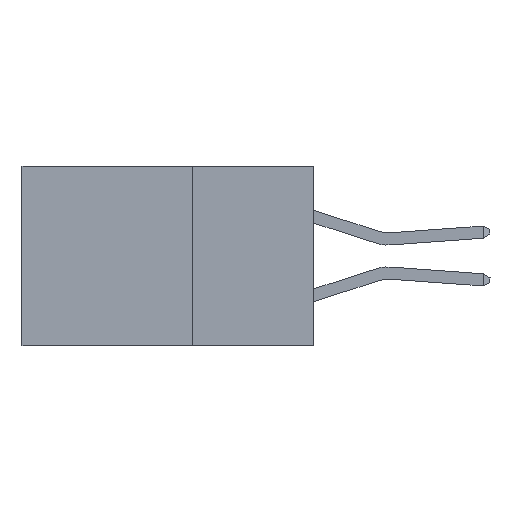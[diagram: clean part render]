
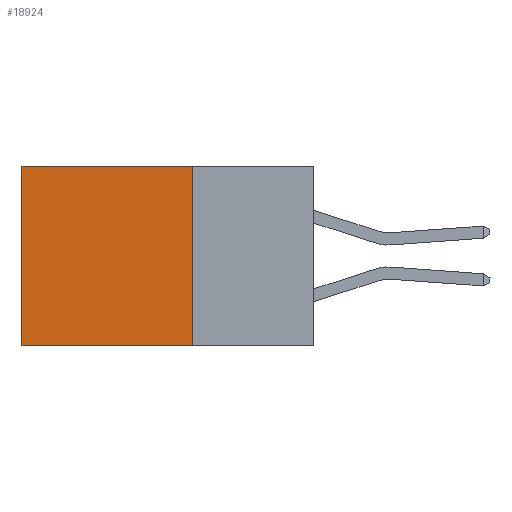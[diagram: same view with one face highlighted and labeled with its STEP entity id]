
A CAD part, left-side view. The second image highlights one B-rep face of the part: STEP entity #18924.
In plain terms, the highlighted planar face has unit normal (-1, 0, 0).
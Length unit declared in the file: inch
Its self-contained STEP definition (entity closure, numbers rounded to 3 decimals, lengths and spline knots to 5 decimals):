
#775 = AXIS2_PLACEMENT_3D ( 'NONE', #8602, #14316, #33722 ) ;
#1108 = DIRECTION ( 'NONE',  ( 0., 1., 0. ) ) ;
#1432 = DIRECTION ( 'NONE',  ( 0., 1., 0. ) ) ;
#2218 = CARTESIAN_POINT ( 'NONE',  ( 0.2875, 0.6, -0.37 ) ) ;
#3618 = EDGE_LOOP ( 'NONE', ( #16414, #12874, #23667, #35190 ) ) ;
#3880 = LINE ( 'NONE', #35024, #18098 ) ;
#6759 = CARTESIAN_POINT ( 'NONE',  ( 0.2875, 0.25, 0. ) ) ;
#6912 = DIRECTION ( 'NONE',  ( 0., 0., -1. ) ) ;
#7972 = CARTESIAN_POINT ( 'NONE',  ( 0.2875, 0.25, -0.37 ) ) ;
#8224 = EDGE_CURVE ( 'NONE', #12353, #23973, #3880, .T. ) ;
#8504 = VECTOR ( 'NONE', #16162, 39.37008 ) ;
#8600 = VECTOR ( 'NONE', #6912, 39.37008 ) ;
#8602 = CARTESIAN_POINT ( 'NONE',  ( 0.2875, 0.25, 0. ) ) ;
#11450 = PLANE ( 'NONE',  #775 ) ;
#12353 = VERTEX_POINT ( 'NONE', #7972 ) ;
#12874 = ORIENTED_EDGE ( 'NONE', *, *, #8224, .F. ) ;
#13288 = CARTESIAN_POINT ( 'NONE',  ( 0.2875, 0.6, 0. ) ) ;
#14132 = VERTEX_POINT ( 'NONE', #25721 ) ;
#14316 = DIRECTION ( 'NONE',  ( 1., 0., 0. ) ) ;
#16162 = DIRECTION ( 'NONE',  ( 0., 0., -1. ) ) ;
#16414 = ORIENTED_EDGE ( 'NONE', *, *, #19381, .T. ) ;
#18098 = VECTOR ( 'NONE', #1432, 39.37008 ) ;
#18575 = VECTOR ( 'NONE', #1108, 39.37008 ) ;
#18924 = ADVANCED_FACE ( 'NONE', ( #24309 ), #11450, .F. ) ;
#19381 = EDGE_CURVE ( 'NONE', #14132, #23973, #24277, .T. ) ;
#23069 = EDGE_CURVE ( 'NONE', #29782, #12353, #31737, .T. ) ;
#23667 = ORIENTED_EDGE ( 'NONE', *, *, #23069, .F. ) ;
#23973 = VERTEX_POINT ( 'NONE', #2218 ) ;
#23997 = CARTESIAN_POINT ( 'NONE',  ( 0.2875, 0.25, 0. ) ) ;
#24277 = LINE ( 'NONE', #13288, #8504 ) ;
#24309 = FACE_OUTER_BOUND ( 'NONE', #3618, .T. ) ;
#25721 = CARTESIAN_POINT ( 'NONE',  ( 0.2875, 0.6, 0. ) ) ;
#25912 = LINE ( 'NONE', #6759, #18575 ) ;
#29209 = CARTESIAN_POINT ( 'NONE',  ( 0.2875, 0.25, 0. ) ) ;
#29782 = VERTEX_POINT ( 'NONE', #23997 ) ;
#31737 = LINE ( 'NONE', #29209, #8600 ) ;
#33510 = EDGE_CURVE ( 'NONE', #29782, #14132, #25912, .T. ) ;
#33722 = DIRECTION ( 'NONE',  ( 0., 0., -1. ) ) ;
#35024 = CARTESIAN_POINT ( 'NONE',  ( 0.2875, 0.25, -0.37 ) ) ;
#35190 = ORIENTED_EDGE ( 'NONE', *, *, #33510, .T. ) ;
